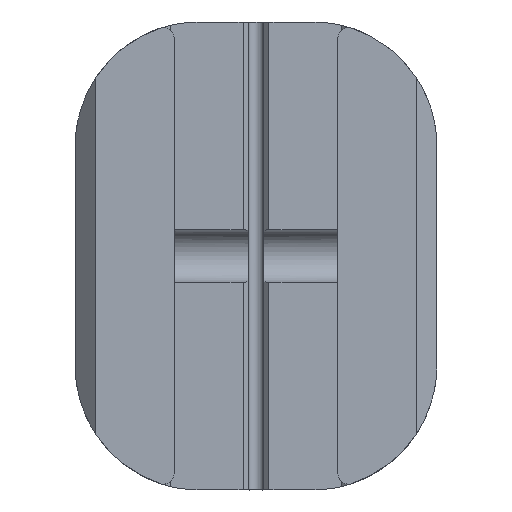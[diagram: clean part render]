
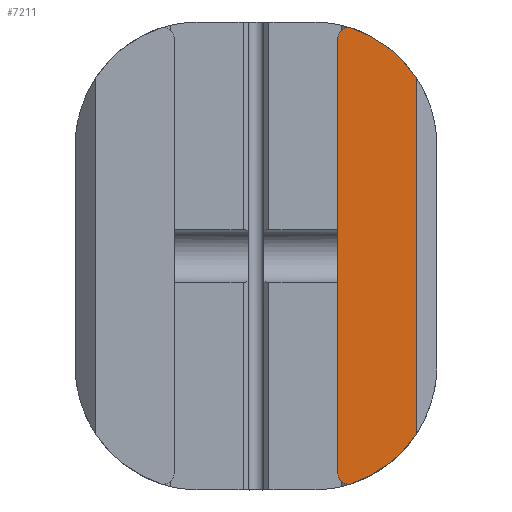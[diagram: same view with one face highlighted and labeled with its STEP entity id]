
A CAD part, top view. The second image highlights one B-rep face of the part: STEP entity #7211.
In plain terms, the highlighted planar face has unit normal (0, 0, 1).
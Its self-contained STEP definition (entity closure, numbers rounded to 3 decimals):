
#127=PLANE('',#8200);
#353=LINE('',#16666,#648);
#374=LINE('',#16737,#669);
#648=VECTOR('',#10204,10.);
#669=VECTOR('',#10265,10.);
#1634=FACE_OUTER_BOUND('',#2137,.T.);
#2137=EDGE_LOOP('',(#6178,#6179,#6180,#6181,#6182,#6183));
#2724=CIRCLE('',#8199,1.);
#2725=CIRCLE('',#8201,1.);
#2726=CIRCLE('',#8202,12.);
#2727=CIRCLE('',#8203,12.);
#3241=VERTEX_POINT('',#16660);
#3243=VERTEX_POINT('',#16664);
#3272=VERTEX_POINT('',#16734);
#3273=VERTEX_POINT('',#16736);
#3306=VERTEX_POINT('',#16840);
#3307=VERTEX_POINT('',#16844);
#4235=EDGE_CURVE('',#3243,#3241,#353,.F.);
#4268=EDGE_CURVE('',#3272,#3273,#374,.T.);
#4322=EDGE_CURVE('',#3306,#3243,#2724,.T.);
#4324=EDGE_CURVE('',#3241,#3307,#2725,.T.);
#4325=EDGE_CURVE('',#3306,#3273,#2726,.T.);
#4326=EDGE_CURVE('',#3272,#3307,#2727,.T.);
#6178=ORIENTED_EDGE('',*,*,#4324,.F.);
#6179=ORIENTED_EDGE('',*,*,#4235,.F.);
#6180=ORIENTED_EDGE('',*,*,#4322,.F.);
#6181=ORIENTED_EDGE('',*,*,#4325,.T.);
#6182=ORIENTED_EDGE('',*,*,#4268,.F.);
#6183=ORIENTED_EDGE('',*,*,#4326,.T.);
#7211=ADVANCED_FACE('',(#1634),#127,.F.);
#8199=AXIS2_PLACEMENT_3D('',#16841,#10373,#10374);
#8200=AXIS2_PLACEMENT_3D('',#16843,#10376,#10377);
#8201=AXIS2_PLACEMENT_3D('',#16845,#10378,#10379);
#8202=AXIS2_PLACEMENT_3D('',#16846,#10380,#10381);
#8203=AXIS2_PLACEMENT_3D('',#16847,#10382,#10383);
#10204=DIRECTION('',(0.,-1.,0.));
#10265=DIRECTION('',(0.,-1.,0.));
#10373=DIRECTION('center_axis',(0.,0.,
-1.));
#10374=DIRECTION('ref_axis',(-0.586,-0.81,0.));
#10376=DIRECTION('center_axis',(0.,0.,
-1.));
#10377=DIRECTION('ref_axis',(-1.,0.,0.));
#10378=DIRECTION('center_axis',(0.,0.,
-1.));
#10379=DIRECTION('ref_axis',(-0.586,0.81,0.));
#10380=DIRECTION('center_axis',(0.,0.,
1.));
#10381=DIRECTION('ref_axis',(1.,0.,0.));
#10382=DIRECTION('center_axis',(0.,0.,
1.));
#10383=DIRECTION('ref_axis',(0.,1.,0.));
#16660=CARTESIAN_POINT('',(7.936,76.102,113.813));
#16664=CARTESIAN_POINT('',(7.936,33.905,113.813));
#16666=CARTESIAN_POINT('',(7.936,67.504,113.813));
#16734=CARTESIAN_POINT('',(15.5,72.286,113.813));
#16736=CARTESIAN_POINT('',(15.5,37.722,113.813));
#16737=CARTESIAN_POINT('',(15.5,40.105,113.813));
#16840=CARTESIAN_POINT('',(9.248,32.955,113.813));
#16841=CARTESIAN_POINT('Origin',(8.936,33.905,113.813));
#16843=CARTESIAN_POINT('Origin',(20.269,40.105,113.813));
#16844=CARTESIAN_POINT('',(9.248,77.052,113.813));
#16845=CARTESIAN_POINT('Origin',(8.936,76.102,113.813));
#16846=CARTESIAN_POINT('Origin',(5.5,44.355,113.813));
#16847=CARTESIAN_POINT('Origin',(5.5,65.653,113.813));
